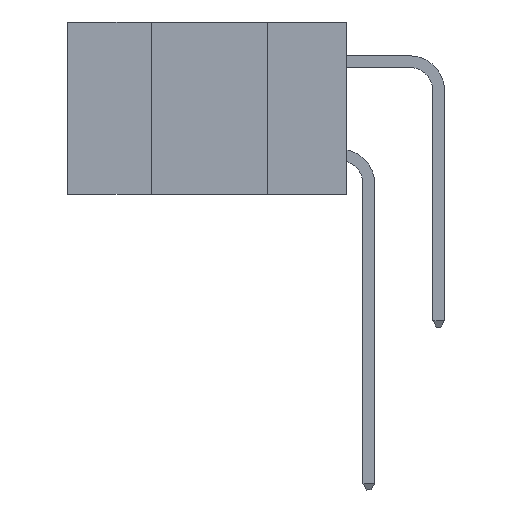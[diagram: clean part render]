
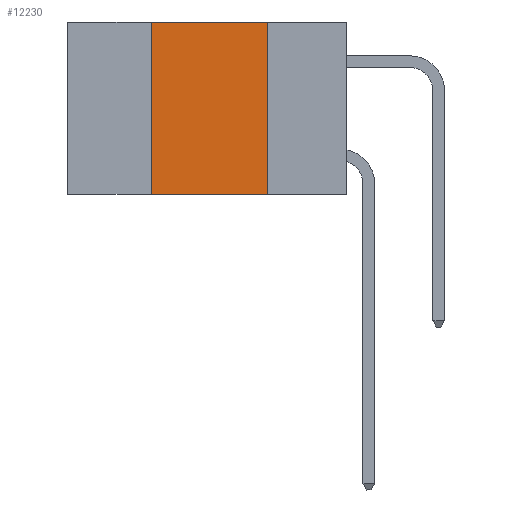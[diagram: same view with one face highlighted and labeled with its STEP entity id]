
A CAD part, left-side view. The second image highlights one B-rep face of the part: STEP entity #12230.
In plain terms, the highlighted planar face has unit normal (-1, 0, 0).
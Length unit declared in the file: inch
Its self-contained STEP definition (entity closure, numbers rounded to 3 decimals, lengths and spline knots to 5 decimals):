
#208 = LINE ( 'NONE', #16250, #16940 ) ;
#640 = DIRECTION ( 'NONE',  ( 0., 0., -1. ) ) ;
#858 = LINE ( 'NONE', #13035, #11182 ) ;
#3119 = DIRECTION ( 'NONE',  ( 0., -1., 0. ) ) ;
#4091 = EDGE_CURVE ( 'NONE', #17018, #9698, #13241, .T. ) ;
#4214 = VERTEX_POINT ( 'NONE', #8973 ) ;
#4347 = AXIS2_PLACEMENT_3D ( 'NONE', #12518, #13808, #5877 ) ;
#5051 = DIRECTION ( 'NONE',  ( 0., -1., 0. ) ) ;
#5549 = DIRECTION ( 'NONE',  ( 0., 0., 1. ) ) ;
#5877 = DIRECTION ( 'NONE',  ( 0., 0., -1. ) ) ;
#5904 = VERTEX_POINT ( 'NONE', #16398 ) ;
#6631 = VECTOR ( 'NONE', #640, 39.37008 ) ;
#6645 = EDGE_CURVE ( 'NONE', #4214, #17018, #858, .T. ) ;
#6847 = EDGE_CURVE ( 'NONE', #5904, #9698, #208, .T. ) ;
#6986 = LINE ( 'NONE', #12214, #16541 ) ;
#7408 = CARTESIAN_POINT ( 'NONE',  ( 0., 0.17, 0. ) ) ;
#8973 = CARTESIAN_POINT ( 'NONE',  ( 0., 0.42, 0. ) ) ;
#9636 = ORIENTED_EDGE ( 'NONE', *, *, #4091, .F. ) ;
#9698 = VERTEX_POINT ( 'NONE', #16689 ) ;
#10020 = ORIENTED_EDGE ( 'NONE', *, *, #6645, .F. ) ;
#11182 = VECTOR ( 'NONE', #5051, 39.37008 ) ;
#11232 = PLANE ( 'NONE',  #4347 ) ;
#11308 = EDGE_CURVE ( 'NONE', #5904, #4214, #6986, .T. ) ;
#12034 = EDGE_LOOP ( 'NONE', ( #9636, #10020, #12522, #13664 ) ) ;
#12214 = CARTESIAN_POINT ( 'NONE',  ( 0., 0.42, 0. ) ) ;
#12230 = ADVANCED_FACE ( 'NONE', ( #15109 ), #11232, .F. ) ;
#12518 = CARTESIAN_POINT ( 'NONE',  ( 0., 0.6, 0. ) ) ;
#12522 = ORIENTED_EDGE ( 'NONE', *, *, #11308, .F. ) ;
#13035 = CARTESIAN_POINT ( 'NONE',  ( 0., 0.6, 0. ) ) ;
#13241 = LINE ( 'NONE', #7408, #6631 ) ;
#13664 = ORIENTED_EDGE ( 'NONE', *, *, #6847, .T. ) ;
#13808 = DIRECTION ( 'NONE',  ( 1., 0., 0. ) ) ;
#15109 = FACE_OUTER_BOUND ( 'NONE', #12034, .T. ) ;
#16250 = CARTESIAN_POINT ( 'NONE',  ( 0., 0.6, -0.37 ) ) ;
#16398 = CARTESIAN_POINT ( 'NONE',  ( 0., 0.42, -0.37 ) ) ;
#16541 = VECTOR ( 'NONE', #5549, 39.37008 ) ;
#16689 = CARTESIAN_POINT ( 'NONE',  ( 0., 0.17, -0.37 ) ) ;
#16802 = CARTESIAN_POINT ( 'NONE',  ( 0., 0.17, 0. ) ) ;
#16940 = VECTOR ( 'NONE', #3119, 39.37008 ) ;
#17018 = VERTEX_POINT ( 'NONE', #16802 ) ;
